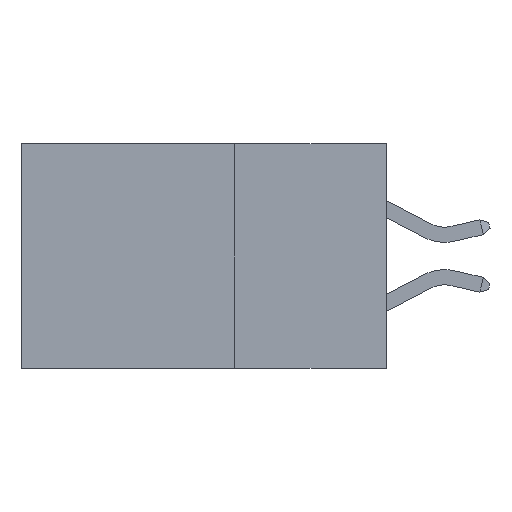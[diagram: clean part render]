
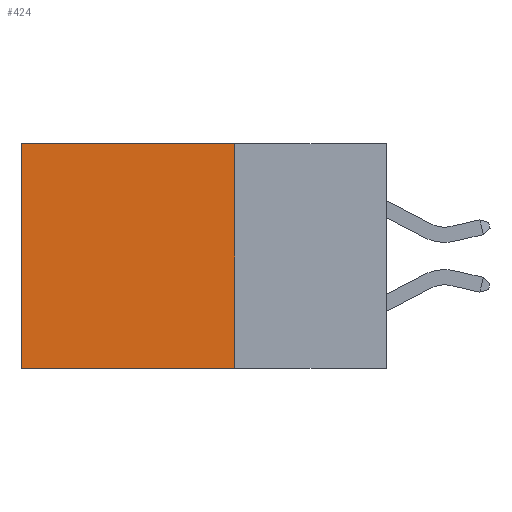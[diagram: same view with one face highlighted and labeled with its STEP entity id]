
A CAD part, left-side view. The second image highlights one B-rep face of the part: STEP entity #424.
In plain terms, the highlighted planar face has unit normal (-1, 0, 0).
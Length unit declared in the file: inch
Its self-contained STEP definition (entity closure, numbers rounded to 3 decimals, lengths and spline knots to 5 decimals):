
#59 = CARTESIAN_POINT ( 'NONE',  ( 0.2615, 0.25, -0.37 ) ) ;
#89 = CARTESIAN_POINT ( 'NONE',  ( 0.2615, 0.25, -0.37 ) ) ;
#164 = CARTESIAN_POINT ( 'NONE',  ( 0.2615, 0.25, 0. ) ) ;
#306 = PLANE ( 'NONE',  #7586 ) ;
#424 = ADVANCED_FACE ( 'NONE', ( #5839 ), #306, .F. ) ;
#487 = CARTESIAN_POINT ( 'NONE',  ( 0.2615, 0.6, -0.37 ) ) ;
#535 = CARTESIAN_POINT ( 'NONE',  ( 0.2615, 0.6, 0. ) ) ;
#1206 = VERTEX_POINT ( 'NONE', #487 ) ;
#1335 = CARTESIAN_POINT ( 'NONE',  ( 0.2615, 0.6, -0.37 ) ) ;
#1346 = EDGE_CURVE ( 'NONE', #3821, #1206, #1927, .T. ) ;
#1358 = DIRECTION ( 'NONE',  ( 0., 0., -1. ) ) ;
#1927 = LINE ( 'NONE', #89, #10591 ) ;
#2117 = LINE ( 'NONE', #4182, #4022 ) ;
#3063 = LINE ( 'NONE', #164, #11193 ) ;
#3145 = CARTESIAN_POINT ( 'NONE',  ( 0.2615, 0.25, 0. ) ) ;
#3208 = DIRECTION ( 'NONE',  ( 0., 0., -1. ) ) ;
#3375 = VERTEX_POINT ( 'NONE', #3145 ) ;
#3462 = EDGE_CURVE ( 'NONE', #11616, #1206, #9925, .T. ) ;
#3752 = DIRECTION ( 'NONE',  ( 0., 1., 0. ) ) ;
#3821 = VERTEX_POINT ( 'NONE', #5314 ) ;
#4022 = VECTOR ( 'NONE', #1358, 39.37008 ) ;
#4182 = CARTESIAN_POINT ( 'NONE',  ( 0.2615, 0.25, -0.37 ) ) ;
#5314 = CARTESIAN_POINT ( 'NONE',  ( 0.2615, 0.25, -0.37 ) ) ;
#5839 = FACE_OUTER_BOUND ( 'NONE', #11850, .T. ) ;
#5966 = VECTOR ( 'NONE', #3208, 39.37008 ) ;
#7586 = AXIS2_PLACEMENT_3D ( 'NONE', #59, #10728, #8733 ) ;
#7964 = ORIENTED_EDGE ( 'NONE', *, *, #3462, .T. ) ;
#8697 = EDGE_CURVE ( 'NONE', #3375, #11616, #3063, .T. ) ;
#8733 = DIRECTION ( 'NONE',  ( 0., 0., -1. ) ) ;
#9039 = DIRECTION ( 'NONE',  ( 0., 1., 0. ) ) ;
#9052 = EDGE_CURVE ( 'NONE', #3375, #3821, #2117, .T. ) ;
#9106 = ORIENTED_EDGE ( 'NONE', *, *, #1346, .F. ) ;
#9925 = LINE ( 'NONE', #1335, #5966 ) ;
#10549 = ORIENTED_EDGE ( 'NONE', *, *, #8697, .T. ) ;
#10591 = VECTOR ( 'NONE', #3752, 39.37008 ) ;
#10728 = DIRECTION ( 'NONE',  ( 1., 0., 0. ) ) ;
#11193 = VECTOR ( 'NONE', #9039, 39.37008 ) ;
#11605 = ORIENTED_EDGE ( 'NONE', *, *, #9052, .F. ) ;
#11616 = VERTEX_POINT ( 'NONE', #535 ) ;
#11850 = EDGE_LOOP ( 'NONE', ( #7964, #9106, #11605, #10549 ) ) ;
